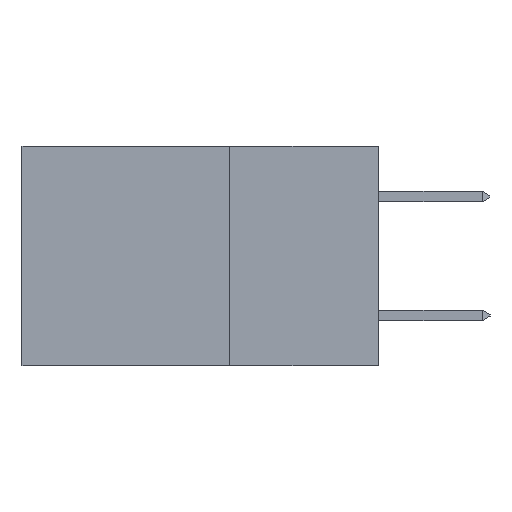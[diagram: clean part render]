
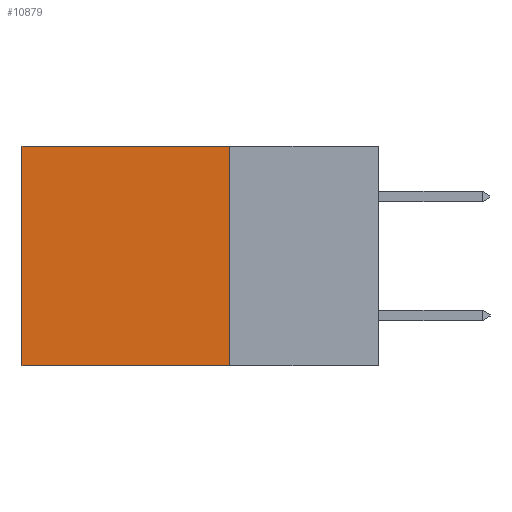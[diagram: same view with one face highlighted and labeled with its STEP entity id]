
A CAD part, left-side view. The second image highlights one B-rep face of the part: STEP entity #10879.
In plain terms, the highlighted planar face has unit normal (-1, 0, 0).
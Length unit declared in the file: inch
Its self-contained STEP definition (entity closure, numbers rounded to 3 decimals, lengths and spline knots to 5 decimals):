
#332 = DIRECTION ( 'NONE',  ( 0., 1., 0. ) ) ;
#888 = EDGE_LOOP ( 'NONE', ( #4537, #12671, #3365, #6895 ) ) ;
#1014 = VECTOR ( 'NONE', #3581, 39.37008 ) ;
#1103 = CARTESIAN_POINT ( 'NONE',  ( 0.2615, 0.25, 0. ) ) ;
#1239 = CARTESIAN_POINT ( 'NONE',  ( 0.2615, 0.6, 0. ) ) ;
#1267 = VERTEX_POINT ( 'NONE', #6742 ) ;
#2108 = EDGE_CURVE ( 'NONE', #3434, #5080, #8798, .T. ) ;
#3365 = ORIENTED_EDGE ( 'NONE', *, *, #11621, .F. ) ;
#3434 = VERTEX_POINT ( 'NONE', #9197 ) ;
#3550 = CARTESIAN_POINT ( 'NONE',  ( 0.2615, 0.25, -0.37 ) ) ;
#3581 = DIRECTION ( 'NONE',  ( 0., 0., -1. ) ) ;
#4537 = ORIENTED_EDGE ( 'NONE', *, *, #8821, .T. ) ;
#4684 = DIRECTION ( 'NONE',  ( 1., 0., 0. ) ) ;
#5080 = VERTEX_POINT ( 'NONE', #1239 ) ;
#5298 = LINE ( 'NONE', #7331, #10684 ) ;
#6509 = AXIS2_PLACEMENT_3D ( 'NONE', #3550, #4684, #12107 ) ;
#6742 = CARTESIAN_POINT ( 'NONE',  ( 0.2615, 0.25, -0.37 ) ) ;
#6895 = ORIENTED_EDGE ( 'NONE', *, *, #2108, .T. ) ;
#7331 = CARTESIAN_POINT ( 'NONE',  ( 0.2615, 0.25, -0.37 ) ) ;
#7600 = LINE ( 'NONE', #11134, #1014 ) ;
#8463 = VECTOR ( 'NONE', #332, 39.37008 ) ;
#8708 = VERTEX_POINT ( 'NONE', #13712 ) ;
#8798 = LINE ( 'NONE', #1103, #8463 ) ;
#8821 = EDGE_CURVE ( 'NONE', #5080, #8708, #12897, .T. ) ;
#9197 = CARTESIAN_POINT ( 'NONE',  ( 0.2615, 0.25, 0. ) ) ;
#9805 = DIRECTION ( 'NONE',  ( 0., 0., -1. ) ) ;
#10073 = PLANE ( 'NONE',  #6509 ) ;
#10185 = VECTOR ( 'NONE', #9805, 39.37008 ) ;
#10684 = VECTOR ( 'NONE', #13579, 39.37008 ) ;
#10841 = CARTESIAN_POINT ( 'NONE',  ( 0.2615, 0.6, -0.37 ) ) ;
#10879 = ADVANCED_FACE ( 'NONE', ( #13011 ), #10073, .F. ) ;
#11134 = CARTESIAN_POINT ( 'NONE',  ( 0.2615, 0.25, -0.37 ) ) ;
#11621 = EDGE_CURVE ( 'NONE', #3434, #1267, #7600, .T. ) ;
#12107 = DIRECTION ( 'NONE',  ( 0., 0., -1. ) ) ;
#12671 = ORIENTED_EDGE ( 'NONE', *, *, #13296, .F. ) ;
#12897 = LINE ( 'NONE', #10841, #10185 ) ;
#13011 = FACE_OUTER_BOUND ( 'NONE', #888, .T. ) ;
#13296 = EDGE_CURVE ( 'NONE', #1267, #8708, #5298, .T. ) ;
#13579 = DIRECTION ( 'NONE',  ( 0., 1., 0. ) ) ;
#13712 = CARTESIAN_POINT ( 'NONE',  ( 0.2615, 0.6, -0.37 ) ) ;
